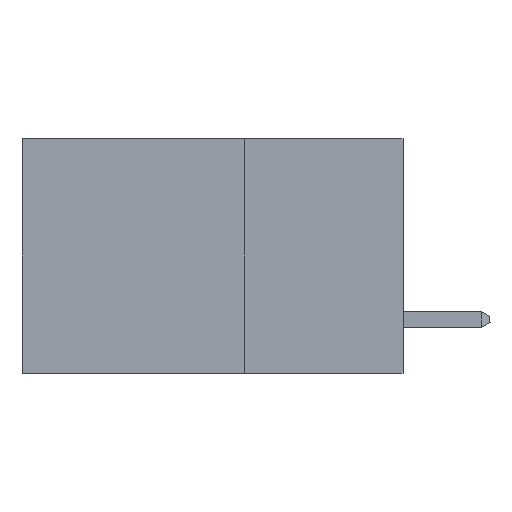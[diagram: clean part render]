
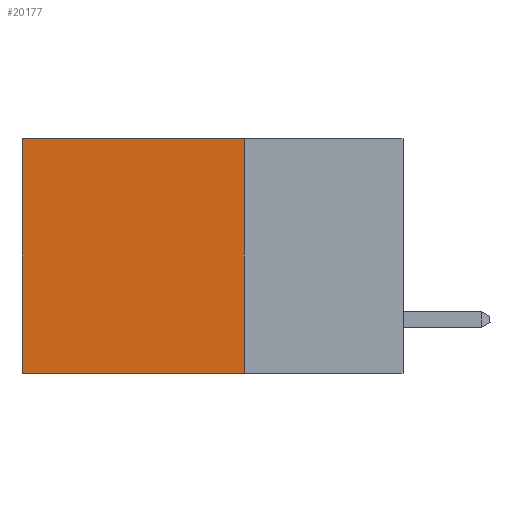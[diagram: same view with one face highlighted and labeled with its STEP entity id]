
A CAD part, left-side view. The second image highlights one B-rep face of the part: STEP entity #20177.
In plain terms, the highlighted planar face has unit normal (-1, 0, 0).
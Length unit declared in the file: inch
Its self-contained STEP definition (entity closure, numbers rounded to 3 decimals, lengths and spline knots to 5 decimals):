
#106 = VECTOR ( 'NONE', #4398, 39.37008 ) ;
#220 = EDGE_CURVE ( 'NONE', #16559, #14969, #11403, .T. ) ;
#744 = CARTESIAN_POINT ( 'NONE',  ( 0.2875, 0.25, 0. ) ) ;
#773 = ORIENTED_EDGE ( 'NONE', *, *, #14568, .T. ) ;
#2528 = EDGE_LOOP ( 'NONE', ( #17112, #18407, #5067, #773 ) ) ;
#2727 = CARTESIAN_POINT ( 'NONE',  ( 0.2875, 0.6, -0.37 ) ) ;
#3567 = LINE ( 'NONE', #7656, #106 ) ;
#3676 = VECTOR ( 'NONE', #8780, 39.37008 ) ;
#4398 = DIRECTION ( 'NONE',  ( 0., 1., 0. ) ) ;
#5067 = ORIENTED_EDGE ( 'NONE', *, *, #220, .F. ) ;
#5568 = VECTOR ( 'NONE', #15116, 39.37008 ) ;
#6521 = PLANE ( 'NONE',  #17629 ) ;
#7656 = CARTESIAN_POINT ( 'NONE',  ( 0.2875, 0.25, -0.37 ) ) ;
#8780 = DIRECTION ( 'NONE',  ( 0., 0., -1. ) ) ;
#9865 = CARTESIAN_POINT ( 'NONE',  ( 0.2875, 0.25, 0. ) ) ;
#10986 = EDGE_CURVE ( 'NONE', #14407, #17657, #13951, .T. ) ;
#11403 = LINE ( 'NONE', #12376, #21072 ) ;
#12376 = CARTESIAN_POINT ( 'NONE',  ( 0.2875, 0.25, 0. ) ) ;
#12591 = DIRECTION ( 'NONE',  ( 0., 0., -1. ) ) ;
#13041 = EDGE_CURVE ( 'NONE', #14969, #17657, #3567, .T. ) ;
#13951 = LINE ( 'NONE', #18495, #3676 ) ;
#14407 = VERTEX_POINT ( 'NONE', #16201 ) ;
#14568 = EDGE_CURVE ( 'NONE', #16559, #14407, #20137, .T. ) ;
#14713 = DIRECTION ( 'NONE',  ( 1., 0., 0. ) ) ;
#14969 = VERTEX_POINT ( 'NONE', #16114 ) ;
#15116 = DIRECTION ( 'NONE',  ( 0., 1., 0. ) ) ;
#16114 = CARTESIAN_POINT ( 'NONE',  ( 0.2875, 0.25, -0.37 ) ) ;
#16201 = CARTESIAN_POINT ( 'NONE',  ( 0.2875, 0.6, 0. ) ) ;
#16559 = VERTEX_POINT ( 'NONE', #19834 ) ;
#17112 = ORIENTED_EDGE ( 'NONE', *, *, #10986, .T. ) ;
#17629 = AXIS2_PLACEMENT_3D ( 'NONE', #9865, #14713, #17859 ) ;
#17657 = VERTEX_POINT ( 'NONE', #2727 ) ;
#17859 = DIRECTION ( 'NONE',  ( 0., 0., -1. ) ) ;
#18407 = ORIENTED_EDGE ( 'NONE', *, *, #13041, .F. ) ;
#18495 = CARTESIAN_POINT ( 'NONE',  ( 0.2875, 0.6, 0. ) ) ;
#19834 = CARTESIAN_POINT ( 'NONE',  ( 0.2875, 0.25, 0. ) ) ;
#20137 = LINE ( 'NONE', #744, #5568 ) ;
#20177 = ADVANCED_FACE ( 'NONE', ( #20374 ), #6521, .F. ) ;
#20374 = FACE_OUTER_BOUND ( 'NONE', #2528, .T. ) ;
#21072 = VECTOR ( 'NONE', #12591, 39.37008 ) ;
